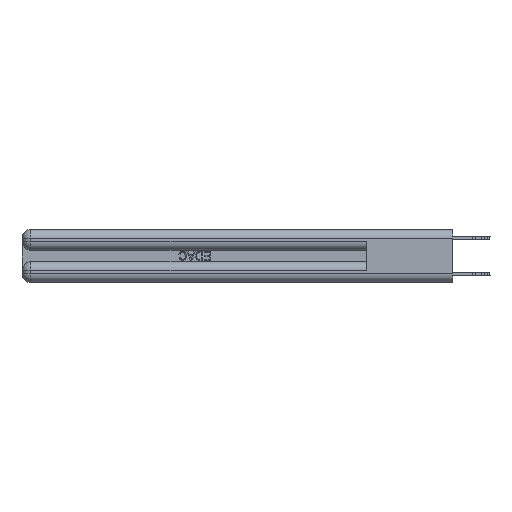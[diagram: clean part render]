
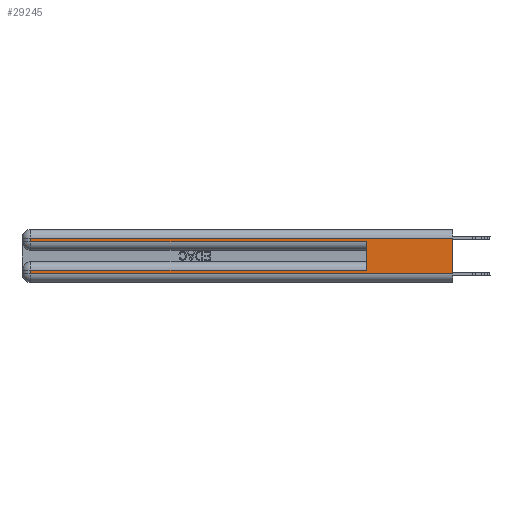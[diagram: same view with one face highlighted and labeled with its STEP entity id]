
A CAD part, left-side view. The second image highlights one B-rep face of the part: STEP entity #29245.
In plain terms, the highlighted planar face has unit normal (-1, 0, 0).
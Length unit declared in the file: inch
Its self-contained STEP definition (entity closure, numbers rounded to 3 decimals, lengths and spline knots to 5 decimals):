
#168 = VERTEX_POINT ( 'NONE', #25362 ) ;
#635 = VERTEX_POINT ( 'NONE', #19748 ) ;
#780 = CARTESIAN_POINT ( 'NONE',  ( 0., 2.94, 0.37 ) ) ;
#1089 = CARTESIAN_POINT ( 'NONE',  ( 0., 0., 0.37 ) ) ;
#1304 = CARTESIAN_POINT ( 'NONE',  ( 0., 2.94, 0.31 ) ) ;
#1320 = DIRECTION ( 'NONE',  ( 0., 0., -1. ) ) ;
#3119 = DIRECTION ( 'NONE',  ( 0., 0., -1. ) ) ;
#3624 = CARTESIAN_POINT ( 'NONE',  ( 0., 0., 0.06 ) ) ;
#3806 = PLANE ( 'NONE',  #11697 ) ;
#3824 = ORIENTED_EDGE ( 'NONE', *, *, #26124, .F. ) ;
#4688 = DIRECTION ( 'NONE',  ( 0., 1., 0. ) ) ;
#4858 = VECTOR ( 'NONE', #27777, 39.37008 ) ;
#5781 = EDGE_CURVE ( 'NONE', #24312, #15019, #31077, .T. ) ;
#5823 = DIRECTION ( 'NONE',  ( 1., 0., 0. ) ) ;
#5853 = LINE ( 'NONE', #16801, #4858 ) ;
#6783 = EDGE_CURVE ( 'NONE', #24312, #635, #24422, .T. ) ;
#7272 = EDGE_CURVE ( 'NONE', #31212, #635, #5853, .T. ) ;
#7782 = VERTEX_POINT ( 'NONE', #3624 ) ;
#8263 = LINE ( 'NONE', #16694, #35520 ) ;
#8306 = CARTESIAN_POINT ( 'NONE',  ( 0., 0., 0.06 ) ) ;
#8324 = ORIENTED_EDGE ( 'NONE', *, *, #13232, .T. ) ;
#8534 = ORIENTED_EDGE ( 'NONE', *, *, #32184, .T. ) ;
#8693 = FACE_OUTER_BOUND ( 'NONE', #29922, .T. ) ;
#8872 = CARTESIAN_POINT ( 'NONE',  ( 0., 0., 0.37 ) ) ;
#11295 = VECTOR ( 'NONE', #4688, 39.37008 ) ;
#11697 = AXIS2_PLACEMENT_3D ( 'NONE', #1089, #5823, #3119 ) ;
#13232 = EDGE_CURVE ( 'NONE', #35122, #31212, #8263, .T. ) ;
#15019 = VERTEX_POINT ( 'NONE', #33570 ) ;
#15449 = CARTESIAN_POINT ( 'NONE',  ( 0., 2.94, 0.285 ) ) ;
#16511 = DIRECTION ( 'NONE',  ( 0., 1., 0. ) ) ;
#16694 = CARTESIAN_POINT ( 'NONE',  ( 0., 2.94, 0.37 ) ) ;
#16801 = CARTESIAN_POINT ( 'NONE',  ( 0., 0., 0.285 ) ) ;
#18147 = VECTOR ( 'NONE', #24833, 39.37008 ) ;
#19394 = CARTESIAN_POINT ( 'NONE',  ( 0., 0., 0.085 ) ) ;
#19748 = CARTESIAN_POINT ( 'NONE',  ( 0., 0.6, 0.285 ) ) ;
#19823 = DIRECTION ( 'NONE',  ( 0., 0., -1. ) ) ;
#20190 = ORIENTED_EDGE ( 'NONE', *, *, #33938, .T. ) ;
#20346 = LINE ( 'NONE', #8872, #31169 ) ;
#20545 = ORIENTED_EDGE ( 'NONE', *, *, #6783, .F. ) ;
#20617 = VECTOR ( 'NONE', #16511, 39.37008 ) ;
#21381 = DIRECTION ( 'NONE',  ( 0., 0., 1. ) ) ;
#22733 = ORIENTED_EDGE ( 'NONE', *, *, #7272, .T. ) ;
#24312 = VERTEX_POINT ( 'NONE', #25605 ) ;
#24422 = LINE ( 'NONE', #32741, #26242 ) ;
#24472 = LINE ( 'NONE', #8306, #18147 ) ;
#24791 = DIRECTION ( 'NONE',  ( 0., 0., -1. ) ) ;
#24833 = DIRECTION ( 'NONE',  ( 0., -1., 0. ) ) ;
#25362 = CARTESIAN_POINT ( 'NONE',  ( 0., 2.94, 0.06 ) ) ;
#25605 = CARTESIAN_POINT ( 'NONE',  ( 0., 0.6, 0.085 ) ) ;
#26061 = LINE ( 'NONE', #29331, #11295 ) ;
#26124 = EDGE_CURVE ( 'NONE', #31930, #7782, #20346, .T. ) ;
#26242 = VECTOR ( 'NONE', #21381, 39.37008 ) ;
#27777 = DIRECTION ( 'NONE',  ( 0., -1., 0. ) ) ;
#29245 = ADVANCED_FACE ( 'NONE', ( #8693 ), #3806, .F. ) ;
#29289 = ORIENTED_EDGE ( 'NONE', *, *, #30130, .T. ) ;
#29331 = CARTESIAN_POINT ( 'NONE',  ( 0., 0., 0.31 ) ) ;
#29922 = EDGE_LOOP ( 'NONE', ( #3824, #20190, #8324, #22733, #20545, #30196, #29289, #8534 ) ) ;
#30130 = EDGE_CURVE ( 'NONE', #15019, #168, #34100, .T. ) ;
#30196 = ORIENTED_EDGE ( 'NONE', *, *, #5781, .T. ) ;
#31077 = LINE ( 'NONE', #19394, #20617 ) ;
#31169 = VECTOR ( 'NONE', #19823, 39.37008 ) ;
#31212 = VERTEX_POINT ( 'NONE', #15449 ) ;
#31930 = VERTEX_POINT ( 'NONE', #33880 ) ;
#32184 = EDGE_CURVE ( 'NONE', #168, #7782, #24472, .T. ) ;
#32741 = CARTESIAN_POINT ( 'NONE',  ( 0., 0.6, 0.145 ) ) ;
#33570 = CARTESIAN_POINT ( 'NONE',  ( 0., 2.94, 0.085 ) ) ;
#33880 = CARTESIAN_POINT ( 'NONE',  ( 0., 0., 0.31 ) ) ;
#33938 = EDGE_CURVE ( 'NONE', #31930, #35122, #26061, .T. ) ;
#34100 = LINE ( 'NONE', #780, #34185 ) ;
#34185 = VECTOR ( 'NONE', #1320, 39.37008 ) ;
#35122 = VERTEX_POINT ( 'NONE', #1304 ) ;
#35520 = VECTOR ( 'NONE', #24791, 39.37008 ) ;
